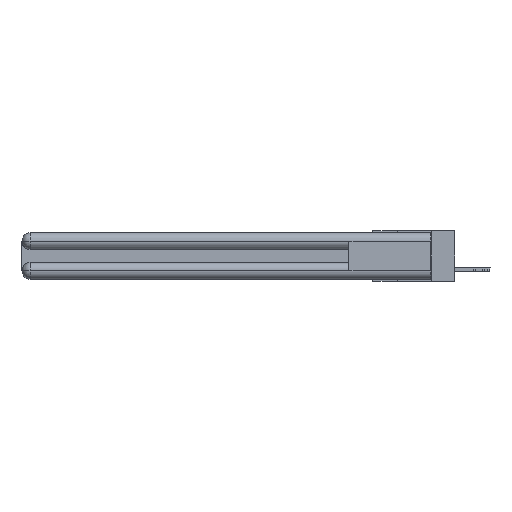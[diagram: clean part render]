
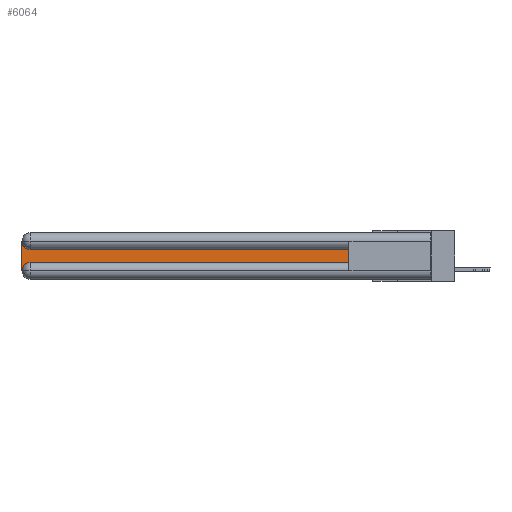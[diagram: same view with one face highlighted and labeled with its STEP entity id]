
A CAD part, left-side view. The second image highlights one B-rep face of the part: STEP entity #6064.
In plain terms, the highlighted planar face has unit normal (-1, 0, 0).
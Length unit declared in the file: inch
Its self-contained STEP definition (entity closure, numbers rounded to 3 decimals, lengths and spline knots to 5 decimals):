
#60 = LINE ( 'NONE', #19487, #27084 ) ;
#1122 = CARTESIAN_POINT ( 'NONE',  ( 0.075, 3., -0.2175 ) ) ;
#2441 = VERTEX_POINT ( 'NONE', #17904 ) ;
#2442 = CARTESIAN_POINT ( 'NONE',  ( 0.075, 3., -0.1225 ) ) ;
#4198 = ORIENTED_EDGE ( 'NONE', *, *, #19312, .T. ) ;
#4489 = LINE ( 'NONE', #20340, #8148 ) ;
#5040 = CARTESIAN_POINT ( 'NONE',  ( 0.075, 2.94, -0.2775 ) ) ;
#5161 = DIRECTION ( 'NONE',  ( 0., 0., -1. ) ) ;
#5706 = VERTEX_POINT ( 'NONE', #12073 ) ;
#6064 = ADVANCED_FACE ( 'NONE', ( #12012 ), #33758, .F. ) ;
#6763 = ORIENTED_EDGE ( 'NONE', *, *, #29869, .T. ) ;
#6845 = DIRECTION ( 'NONE',  ( 0., 1., 0. ) ) ;
#7773 = DIRECTION ( 'NONE',  ( 0., 0., -1. ) ) ;
#8148 = VECTOR ( 'NONE', #6845, 39.37008 ) ;
#8871 = VERTEX_POINT ( 'NONE', #27073 ) ;
#8981 = EDGE_CURVE ( 'NONE', #22615, #22478, #15050, .T. ) ;
#10196 = CARTESIAN_POINT ( 'NONE',  ( 0.075, 0.6, -0.1225 ) ) ;
#11414 = AXIS2_PLACEMENT_3D ( 'NONE', #25315, #31053, #28866 ) ;
#11960 = CARTESIAN_POINT ( 'NONE',  ( 0.075, 3., -0.0625 ) ) ;
#12012 = FACE_OUTER_BOUND ( 'NONE', #26989, .T. ) ;
#12073 = CARTESIAN_POINT ( 'NONE',  ( 0.075, 2.94, -0.2175 ) ) ;
#12409 = ORIENTED_EDGE ( 'NONE', *, *, #27633, .T. ) ;
#14510 = VECTOR ( 'NONE', #16518, 39.37008 ) ;
#14584 = VERTEX_POINT ( 'NONE', #10196 ) ;
#14676 = AXIS2_PLACEMENT_3D ( 'NONE', #2442, #15509, #5161 ) ;
#14822 = CARTESIAN_POINT ( 'NONE',  ( 0.075, 0.6, -0.2175 ) ) ;
#15050 = CIRCLE ( 'NONE', #11414, 0.06 ) ;
#15247 = EDGE_CURVE ( 'NONE', #8871, #5706, #24039, .T. ) ;
#15509 = DIRECTION ( 'NONE',  ( 1., 0., 0. ) ) ;
#16349 = LINE ( 'NONE', #14822, #24971 ) ;
#16518 = DIRECTION ( 'NONE',  ( 0., 0., -1. ) ) ;
#16551 = ORIENTED_EDGE ( 'NONE', *, *, #17235, .T. ) ;
#16825 = ORIENTED_EDGE ( 'NONE', *, *, #8981, .T. ) ;
#17235 = EDGE_CURVE ( 'NONE', #14584, #22615, #4489, .T. ) ;
#17577 = DIRECTION ( 'NONE',  ( 0., 0., 1. ) ) ;
#17904 = CARTESIAN_POINT ( 'NONE',  ( 0.075, 0.6, -0.2175 ) ) ;
#19312 = EDGE_CURVE ( 'NONE', #22478, #8871, #23157, .T. ) ;
#19487 = CARTESIAN_POINT ( 'NONE',  ( 0.075, 0.6, -0.2175 ) ) ;
#20340 = CARTESIAN_POINT ( 'NONE',  ( 0.075, 0.6, -0.1225 ) ) ;
#22099 = DIRECTION ( 'NONE',  ( 0., -1., 0. ) ) ;
#22478 = VERTEX_POINT ( 'NONE', #11960 ) ;
#22615 = VERTEX_POINT ( 'NONE', #22628 ) ;
#22628 = CARTESIAN_POINT ( 'NONE',  ( 0.075, 2.94, -0.1225 ) ) ;
#23157 = LINE ( 'NONE', #1122, #14510 ) ;
#24039 = CIRCLE ( 'NONE', #24539, 0.06 ) ;
#24539 = AXIS2_PLACEMENT_3D ( 'NONE', #5040, #31453, #7773 ) ;
#24971 = VECTOR ( 'NONE', #17577, 39.37008 ) ;
#25315 = CARTESIAN_POINT ( 'NONE',  ( 0.075, 2.94, -0.0625 ) ) ;
#26989 = EDGE_LOOP ( 'NONE', ( #16551, #16825, #4198, #30737, #6763, #12409 ) ) ;
#27073 = CARTESIAN_POINT ( 'NONE',  ( 0.075, 3., -0.2775 ) ) ;
#27084 = VECTOR ( 'NONE', #22099, 39.37008 ) ;
#27633 = EDGE_CURVE ( 'NONE', #2441, #14584, #16349, .T. ) ;
#28866 = DIRECTION ( 'NONE',  ( 0., 0., -1. ) ) ;
#29869 = EDGE_CURVE ( 'NONE', #5706, #2441, #60, .T. ) ;
#30737 = ORIENTED_EDGE ( 'NONE', *, *, #15247, .T. ) ;
#31053 = DIRECTION ( 'NONE',  ( 1., 0., 0. ) ) ;
#31453 = DIRECTION ( 'NONE',  ( 1., 0., 0. ) ) ;
#33758 = PLANE ( 'NONE',  #14676 ) ;
